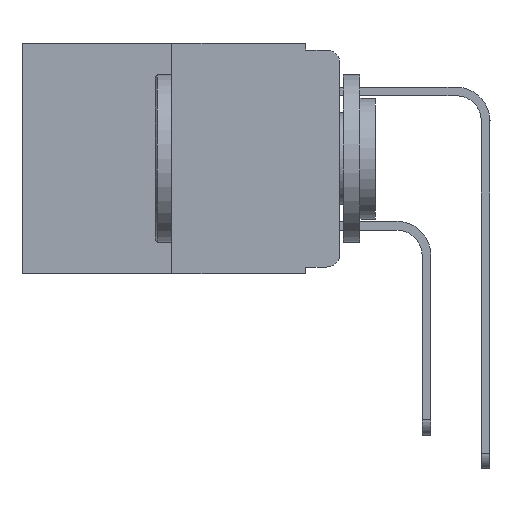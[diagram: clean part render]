
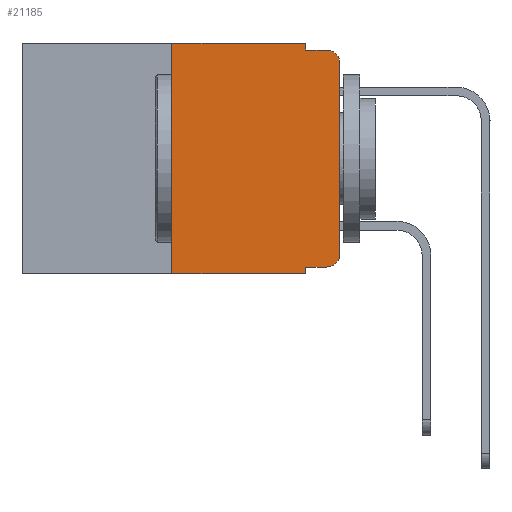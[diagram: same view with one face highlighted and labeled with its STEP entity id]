
A CAD part, left-side view. The second image highlights one B-rep face of the part: STEP entity #21185.
In plain terms, the highlighted planar face has unit normal (-1, 0, 0).
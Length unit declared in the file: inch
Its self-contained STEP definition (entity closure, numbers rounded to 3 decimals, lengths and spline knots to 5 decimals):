
#60 = EDGE_CURVE ( 'NONE', #9766, #9315, #14065, .T. ) ;
#312 = AXIS2_PLACEMENT_3D ( 'NONE', #23321, #19294, #6673 ) ;
#1201 = EDGE_LOOP ( 'NONE', ( #9323, #15565, #26544, #16880, #18870, #3342, #14614, #10340, #23380, #8012 ) ) ;
#1519 = LINE ( 'NONE', #23898, #11569 ) ;
#1700 = VERTEX_POINT ( 'NONE', #5527 ) ;
#2144 = DIRECTION ( 'NONE',  ( 0., -1., 0. ) ) ;
#2172 = VERTEX_POINT ( 'NONE', #15568 ) ;
#2654 = VERTEX_POINT ( 'NONE', #16597 ) ;
#3342 = ORIENTED_EDGE ( 'NONE', *, *, #18240, .F. ) ;
#3537 = EDGE_CURVE ( 'NONE', #9587, #2172, #15230, .T. ) ;
#4383 = AXIS2_PLACEMENT_3D ( 'NONE', #18299, #5660, #20370 ) ;
#4745 = VECTOR ( 'NONE', #7510, 39.37008 ) ;
#5047 = LINE ( 'NONE', #20545, #10712 ) ;
#5527 = CARTESIAN_POINT ( 'NONE',  ( 0., 0.25, -0.343 ) ) ;
#5658 = CIRCLE ( 'NONE', #4383, 0.02 ) ;
#5660 = DIRECTION ( 'NONE',  ( -1., 0., 0. ) ) ;
#5748 = VECTOR ( 'NONE', #2144, 39.37008 ) ;
#5829 = DIRECTION ( 'NONE',  ( 0., -1., 0. ) ) ;
#6400 = CARTESIAN_POINT ( 'NONE',  ( 0., 0.473, 0. ) ) ;
#6673 = DIRECTION ( 'NONE',  ( 0., 0., -1. ) ) ;
#7050 = CARTESIAN_POINT ( 'NONE',  ( 0., 0.25, 0. ) ) ;
#7192 = CARTESIAN_POINT ( 'NONE',  ( 0., 0.02, -0.333 ) ) ;
#7510 = DIRECTION ( 'NONE',  ( 0., -1., 0. ) ) ;
#7679 = CARTESIAN_POINT ( 'NONE',  ( 0., 0., -0.313 ) ) ;
#8012 = ORIENTED_EDGE ( 'NONE', *, *, #60, .T. ) ;
#9085 = LINE ( 'NONE', #15096, #24394 ) ;
#9103 = VECTOR ( 'NONE', #9189, 39.37008 ) ;
#9189 = DIRECTION ( 'NONE',  ( 0., 0., 1. ) ) ;
#9311 = VERTEX_POINT ( 'NONE', #16032 ) ;
#9315 = VERTEX_POINT ( 'NONE', #7679 ) ;
#9323 = ORIENTED_EDGE ( 'NONE', *, *, #24060, .T. ) ;
#9587 = VERTEX_POINT ( 'NONE', #12939 ) ;
#9766 = VERTEX_POINT ( 'NONE', #7192 ) ;
#9778 = EDGE_CURVE ( 'NONE', #9311, #12610, #1519, .T. ) ;
#10340 = ORIENTED_EDGE ( 'NONE', *, *, #3537, .F. ) ;
#10485 = CARTESIAN_POINT ( 'NONE',  ( 0., 0.051, 0. ) ) ;
#10712 = VECTOR ( 'NONE', #5829, 39.37008 ) ;
#10996 = DIRECTION ( 'NONE',  ( 0., -1., 0. ) ) ;
#11094 = LINE ( 'NONE', #18020, #4745 ) ;
#11453 = VERTEX_POINT ( 'NONE', #24348 ) ;
#11569 = VECTOR ( 'NONE', #25950, 39.37008 ) ;
#12089 = EDGE_CURVE ( 'NONE', #9587, #9766, #11094, .T. ) ;
#12610 = VERTEX_POINT ( 'NONE', #24681 ) ;
#12709 = LINE ( 'NONE', #6400, #5748 ) ;
#12939 = CARTESIAN_POINT ( 'NONE',  ( 0., 0.051, -0.333 ) ) ;
#13462 = AXIS2_PLACEMENT_3D ( 'NONE', #22606, #17352, #17471 ) ;
#14065 = CIRCLE ( 'NONE', #13462, 0.02 ) ;
#14182 = CARTESIAN_POINT ( 'NONE',  ( 0., 0.25, 0. ) ) ;
#14585 = VECTOR ( 'NONE', #25013, 39.37008 ) ;
#14614 = ORIENTED_EDGE ( 'NONE', *, *, #25177, .T. ) ;
#15096 = CARTESIAN_POINT ( 'NONE',  ( 0., 0.473, -0.343 ) ) ;
#15205 = EDGE_CURVE ( 'NONE', #2654, #11453, #5658, .T. ) ;
#15230 = LINE ( 'NONE', #10485, #14585 ) ;
#15565 = ORIENTED_EDGE ( 'NONE', *, *, #15205, .T. ) ;
#15568 = CARTESIAN_POINT ( 'NONE',  ( 0., 0.051, -0.343 ) ) ;
#16032 = CARTESIAN_POINT ( 'NONE',  ( 0., 0.051, 0. ) ) ;
#16597 = CARTESIAN_POINT ( 'NONE',  ( 0., 0., -0.03 ) ) ;
#16880 = ORIENTED_EDGE ( 'NONE', *, *, #9778, .F. ) ;
#17169 = PLANE ( 'NONE',  #312 ) ;
#17352 = DIRECTION ( 'NONE',  ( -1., 0., 0. ) ) ;
#17471 = DIRECTION ( 'NONE',  ( 0., 0., -1. ) ) ;
#18020 = CARTESIAN_POINT ( 'NONE',  ( 0., 0.051, -0.333 ) ) ;
#18240 = EDGE_CURVE ( 'NONE', #1700, #22670, #26829, .T. ) ;
#18299 = CARTESIAN_POINT ( 'NONE',  ( 0., 0.02, -0.03 ) ) ;
#18870 = ORIENTED_EDGE ( 'NONE', *, *, #21130, .F. ) ;
#19294 = DIRECTION ( 'NONE',  ( 1., 0., 0. ) ) ;
#19646 = DIRECTION ( 'NONE',  ( 0., 0., 1. ) ) ;
#20370 = DIRECTION ( 'NONE',  ( 0., 0., -1. ) ) ;
#20545 = CARTESIAN_POINT ( 'NONE',  ( 0., 0.051, -0.01 ) ) ;
#20552 = FACE_OUTER_BOUND ( 'NONE', #1201, .T. ) ;
#21130 = EDGE_CURVE ( 'NONE', #22670, #9311, #12709, .T. ) ;
#21185 = ADVANCED_FACE ( 'NONE', ( #20552 ), #17169, .F. ) ;
#22606 = CARTESIAN_POINT ( 'NONE',  ( 0., 0.02, -0.313 ) ) ;
#22670 = VERTEX_POINT ( 'NONE', #14182 ) ;
#23321 = CARTESIAN_POINT ( 'NONE',  ( 0., 0.473, 0. ) ) ;
#23380 = ORIENTED_EDGE ( 'NONE', *, *, #12089, .T. ) ;
#23776 = CARTESIAN_POINT ( 'NONE',  ( 0., 0., 0. ) ) ;
#23898 = CARTESIAN_POINT ( 'NONE',  ( 0., 0.051, 0. ) ) ;
#24060 = EDGE_CURVE ( 'NONE', #9315, #2654, #25691, .T. ) ;
#24348 = CARTESIAN_POINT ( 'NONE',  ( 0., 0.02, -0.01 ) ) ;
#24394 = VECTOR ( 'NONE', #10996, 39.37008 ) ;
#24681 = CARTESIAN_POINT ( 'NONE',  ( 0., 0.051, -0.01 ) ) ;
#25013 = DIRECTION ( 'NONE',  ( 0., 0., -1. ) ) ;
#25177 = EDGE_CURVE ( 'NONE', #1700, #2172, #9085, .T. ) ;
#25691 = LINE ( 'NONE', #23776, #9103 ) ;
#25950 = DIRECTION ( 'NONE',  ( 0., 0., -1. ) ) ;
#26188 = VECTOR ( 'NONE', #19646, 39.37008 ) ;
#26544 = ORIENTED_EDGE ( 'NONE', *, *, #26974, .F. ) ;
#26829 = LINE ( 'NONE', #7050, #26188 ) ;
#26974 = EDGE_CURVE ( 'NONE', #12610, #11453, #5047, .T. ) ;
